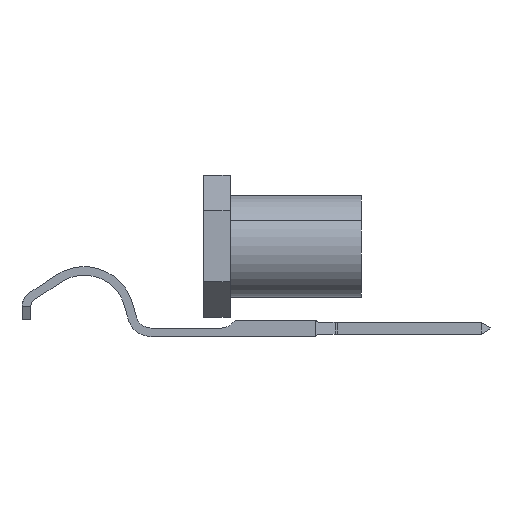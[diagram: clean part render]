
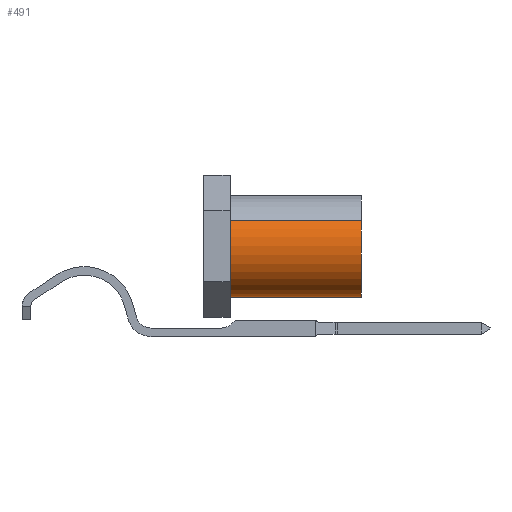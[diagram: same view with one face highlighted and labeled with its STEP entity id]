
A CAD part, left-side view. The second image highlights one B-rep face of the part: STEP entity #491.
In plain terms, the highlighted cylindrical face has radius 1.968 mm (diameter 3.937 mm), a partial arc.
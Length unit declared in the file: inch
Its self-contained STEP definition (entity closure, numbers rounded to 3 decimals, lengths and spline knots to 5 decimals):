
#4 = VERTEX_POINT ( 'NONE', #1688 ) ;
#26 = DIRECTION ( 'NONE',  ( 0., -1., 0. ) ) ;
#212 = DIRECTION ( 'NONE',  ( 0., 0., 1. ) ) ;
#215 = DIRECTION ( 'NONE',  ( 0., 1., 0. ) ) ;
#245 = CARTESIAN_POINT ( 'NONE',  ( 0., 0.04, 0. ) ) ;
#321 = VERTEX_POINT ( 'NONE', #7256 ) ;
#491 = ADVANCED_FACE ( 'NONE', ( #6969 ), #6941, .T. ) ;
#811 = DIRECTION ( 'NONE',  ( 0., 0., 1. ) ) ;
#988 = CARTESIAN_POINT ( 'NONE',  ( 0., 0.24, 0.0775 ) ) ;
#1218 = EDGE_LOOP ( 'NONE', ( #6051, #6127, #6422, #6697 ) ) ;
#1688 = CARTESIAN_POINT ( 'NONE',  ( 0., 0.04, 0.0775 ) ) ;
#1707 = AXIS2_PLACEMENT_3D ( 'NONE', #7590, #7573, #811 ) ;
#1861 = DIRECTION ( 'NONE',  ( 0., -1., 0. ) ) ;
#1897 = CIRCLE ( 'NONE', #2528, 0.0775 ) ;
#2111 = CARTESIAN_POINT ( 'NONE',  ( 0., 0.24, -0.0775 ) ) ;
#2528 = AXIS2_PLACEMENT_3D ( 'NONE', #245, #215, #212 ) ;
#2630 = VERTEX_POINT ( 'NONE', #988 ) ;
#3856 = DIRECTION ( 'NONE',  ( 0., -1., 0. ) ) ;
#4289 = VERTEX_POINT ( 'NONE', #5351 ) ;
#4318 = AXIS2_PLACEMENT_3D ( 'NONE', #8312, #26, #8168 ) ;
#4472 = CARTESIAN_POINT ( 'NONE',  ( 0., 0.24, 0.0775 ) ) ;
#4887 = CIRCLE ( 'NONE', #1707, 0.0775 ) ;
#5351 = CARTESIAN_POINT ( 'NONE',  ( 0., 0.24, -0.0775 ) ) ;
#5433 = EDGE_CURVE ( 'NONE', #321, #4, #1897, .T. ) ;
#5822 = EDGE_CURVE ( 'NONE', #4289, #2630, #4887, .T. ) ;
#6051 = ORIENTED_EDGE ( 'NONE', *, *, #7640, .F. ) ;
#6127 = ORIENTED_EDGE ( 'NONE', *, *, #5822, .F. ) ;
#6422 = ORIENTED_EDGE ( 'NONE', *, *, #6470, .T. ) ;
#6470 = EDGE_CURVE ( 'NONE', #4289, #321, #8036, .T. ) ;
#6697 = ORIENTED_EDGE ( 'NONE', *, *, #5433, .T. ) ;
#6941 = CYLINDRICAL_SURFACE ( 'NONE', #4318, 0.0775 ) ;
#6969 = FACE_OUTER_BOUND ( 'NONE', #1218, .T. ) ;
#7256 = CARTESIAN_POINT ( 'NONE',  ( 0., 0.04, -0.0775 ) ) ;
#7573 = DIRECTION ( 'NONE',  ( 0., 1., 0. ) ) ;
#7590 = CARTESIAN_POINT ( 'NONE',  ( 0., 0.24, 0. ) ) ;
#7640 = EDGE_CURVE ( 'NONE', #2630, #4, #8161, .T. ) ;
#7738 = VECTOR ( 'NONE', #1861, 39.37008 ) ;
#8036 = LINE ( 'NONE', #2111, #7738 ) ;
#8161 = LINE ( 'NONE', #4472, #8173 ) ;
#8168 = DIRECTION ( 'NONE',  ( 0., 0., -1. ) ) ;
#8173 = VECTOR ( 'NONE', #3856, 39.37008 ) ;
#8312 = CARTESIAN_POINT ( 'NONE',  ( 0., 0.24, 0. ) ) ;
